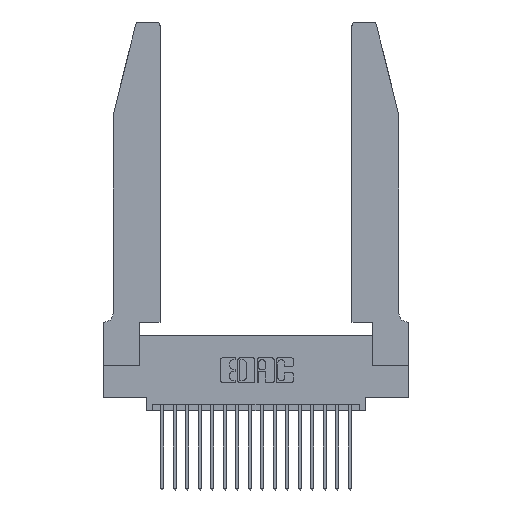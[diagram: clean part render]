
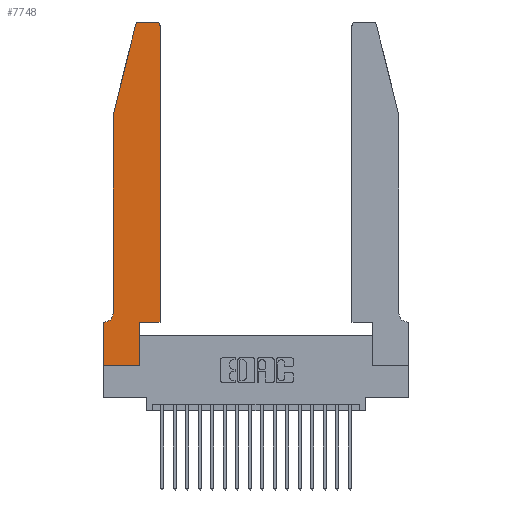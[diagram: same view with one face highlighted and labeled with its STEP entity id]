
A CAD part, top view. The second image highlights one B-rep face of the part: STEP entity #7748.
In plain terms, the highlighted planar face has unit normal (0, 0, 1).
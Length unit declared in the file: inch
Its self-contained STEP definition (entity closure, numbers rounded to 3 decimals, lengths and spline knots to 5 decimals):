
#92 = CARTESIAN_POINT ( 'NONE',  ( 0.2605, 2.75, 0.37 ) ) ;
#198 = DIRECTION ( 'NONE',  ( -1., 0., 0. ) ) ;
#615 = CARTESIAN_POINT ( 'NONE',  ( 0.4505, 0.35, 0.37 ) ) ;
#649 = ORIENTED_EDGE ( 'NONE', *, *, #16710, .T. ) ;
#1823 = VERTEX_POINT ( 'NONE', #10406 ) ;
#1873 = VERTEX_POINT ( 'NONE', #13805 ) ;
#2402 = VERTEX_POINT ( 'NONE', #5534 ) ;
#2595 = CARTESIAN_POINT ( 'NONE',  ( 0.25487, 2.72718, 0.37 ) ) ;
#2842 = DIRECTION ( 'NONE',  ( 0., 0., 1. ) ) ;
#2974 = CARTESIAN_POINT ( 'NONE',  ( 0., 0., 0.37 ) ) ;
#3159 = EDGE_CURVE ( 'NONE', #13457, #8409, #9979, .T. ) ;
#3183 = CARTESIAN_POINT ( 'NONE',  ( 0.0055, 0.35, 0.37 ) ) ;
#3323 = FACE_OUTER_BOUND ( 'NONE', #18775, .T. ) ;
#3394 = LINE ( 'NONE', #15397, #6184 ) ;
#3565 = CIRCLE ( 'NONE', #10356, 0.07 ) ;
#3956 = DIRECTION ( 'NONE',  ( 0., 1., 0. ) ) ;
#4729 = VERTEX_POINT ( 'NONE', #3183 ) ;
#5154 = EDGE_CURVE ( 'NONE', #2402, #15392, #16487, .T. ) ;
#5311 = EDGE_CURVE ( 'NONE', #18256, #2402, #11683, .T. ) ;
#5534 = CARTESIAN_POINT ( 'NONE',  ( 0.284, 2.75, 0.37 ) ) ;
#6184 = VECTOR ( 'NONE', #3956, 39.37008 ) ;
#6278 = DIRECTION ( 'NONE',  ( 0., 0., 1. ) ) ;
#6350 = CARTESIAN_POINT ( 'NONE',  ( 0.284, 2.72, 0.37 ) ) ;
#6477 = ORIENTED_EDGE ( 'NONE', *, *, #20467, .T. ) ;
#6614 = EDGE_CURVE ( 'NONE', #8911, #20233, #6688, .T. ) ;
#6688 = LINE ( 'NONE', #12629, #11731 ) ;
#6787 = ORIENTED_EDGE ( 'NONE', *, *, #10828, .T. ) ;
#7093 = CARTESIAN_POINT ( 'NONE',  ( 0.4205, 2.72, 0.37 ) ) ;
#7231 = CARTESIAN_POINT ( 'NONE',  ( 0.4205, 2.75, 0.37 ) ) ;
#7325 = DIRECTION ( 'NONE',  ( -1., 0., 0. ) ) ;
#7343 = EDGE_CURVE ( 'NONE', #20233, #1823, #18026, .T. ) ;
#7470 = ORIENTED_EDGE ( 'NONE', *, *, #7343, .T. ) ;
#7748 = ADVANCED_FACE ( 'NONE', ( #3323 ), #11911, .T. ) ;
#7940 = VECTOR ( 'NONE', #198, 39.37008 ) ;
#8409 = VERTEX_POINT ( 'NONE', #8895 ) ;
#8895 = CARTESIAN_POINT ( 'NONE',  ( 0.0755, 0.42, 0.37 ) ) ;
#8911 = VERTEX_POINT ( 'NONE', #19787 ) ;
#9188 = DIRECTION ( 'NONE',  ( 1., 0., 0. ) ) ;
#9719 = ORIENTED_EDGE ( 'NONE', *, *, #6614, .T. ) ;
#9979 = LINE ( 'NONE', #15523, #20868 ) ;
#10356 = AXIS2_PLACEMENT_3D ( 'NONE', #20347, #12143, #7325 ) ;
#10406 = CARTESIAN_POINT ( 'NONE',  ( 0.2865, 0., 0.37 ) ) ;
#10728 = DIRECTION ( 'NONE',  ( 0., -1., 0. ) ) ;
#10732 = VERTEX_POINT ( 'NONE', #17346 ) ;
#10793 = EDGE_CURVE ( 'NONE', #1873, #18256, #17385, .T. ) ;
#10828 = EDGE_CURVE ( 'NONE', #1823, #10732, #19160, .T. ) ;
#11485 = ORIENTED_EDGE ( 'NONE', *, *, #5311, .T. ) ;
#11492 = DIRECTION ( 'NONE',  ( -1., 0., 0. ) ) ;
#11619 = ORIENTED_EDGE ( 'NONE', *, *, #14231, .T. ) ;
#11683 = LINE ( 'NONE', #92, #18528 ) ;
#11731 = VECTOR ( 'NONE', #16290, 39.37008 ) ;
#11852 = AXIS2_PLACEMENT_3D ( 'NONE', #16579, #2842, #9188 ) ;
#11896 = DIRECTION ( 'NONE',  ( 1., 0., 0. ) ) ;
#11911 = PLANE ( 'NONE',  #11852 ) ;
#12005 = DIRECTION ( 'NONE',  ( 1., 0., 0. ) ) ;
#12143 = DIRECTION ( 'NONE',  ( 0., 0., -1. ) ) ;
#12629 = CARTESIAN_POINT ( 'NONE',  ( 0., 0., 0.37 ) ) ;
#13005 = CARTESIAN_POINT ( 'NONE',  ( 0.4505, 0.35, 0.37 ) ) ;
#13352 = CARTESIAN_POINT ( 'NONE',  ( 0.0755, 2., 0.37 ) ) ;
#13457 = VERTEX_POINT ( 'NONE', #16634 ) ;
#13805 = CARTESIAN_POINT ( 'NONE',  ( 0.4505, 2.72, 0.37 ) ) ;
#13833 = VECTOR ( 'NONE', #18332, 39.37008 ) ;
#14231 = EDGE_CURVE ( 'NONE', #15392, #13457, #19196, .T. ) ;
#14837 = CARTESIAN_POINT ( 'NONE',  ( 0.0755, 0.35, 0.37 ) ) ;
#15274 = ORIENTED_EDGE ( 'NONE', *, *, #10793, .T. ) ;
#15392 = VERTEX_POINT ( 'NONE', #2595 ) ;
#15397 = CARTESIAN_POINT ( 'NONE',  ( 0.4505, 0.35, 0.37 ) ) ;
#15523 = CARTESIAN_POINT ( 'NONE',  ( 0.0755, 2., 0.37 ) ) ;
#15713 = CARTESIAN_POINT ( 'NONE',  ( 0., 0., 0.37 ) ) ;
#16290 = DIRECTION ( 'NONE',  ( 0., -1., 0. ) ) ;
#16487 = CIRCLE ( 'NONE', #16822, 0.03 ) ;
#16579 = CARTESIAN_POINT ( 'NONE',  ( 0., 0.35, 0.37 ) ) ;
#16634 = CARTESIAN_POINT ( 'NONE',  ( 0.0755, 2., 0.37 ) ) ;
#16701 = CARTESIAN_POINT ( 'NONE',  ( 0.2865, 0.35, 0.37 ) ) ;
#16710 = EDGE_CURVE ( 'NONE', #10732, #19386, #18593, .T. ) ;
#16822 = AXIS2_PLACEMENT_3D ( 'NONE', #6350, #6278, #17587 ) ;
#17293 = LINE ( 'NONE', #14837, #7940 ) ;
#17346 = CARTESIAN_POINT ( 'NONE',  ( 0.2865, 0.35, 0.37 ) ) ;
#17385 = CIRCLE ( 'NONE', #20580, 0.03 ) ;
#17531 = EDGE_CURVE ( 'NONE', #4729, #8911, #17293, .T. ) ;
#17587 = DIRECTION ( 'NONE',  ( 1., 0., 0. ) ) ;
#17596 = DIRECTION ( 'NONE',  ( -0.239, -0.971, 0. ) ) ;
#17795 = ORIENTED_EDGE ( 'NONE', *, *, #19012, .T. ) ;
#18026 = LINE ( 'NONE', #15713, #20314 ) ;
#18256 = VERTEX_POINT ( 'NONE', #7231 ) ;
#18332 = DIRECTION ( 'NONE',  ( 0., 1., 0. ) ) ;
#18348 = ORIENTED_EDGE ( 'NONE', *, *, #5154, .T. ) ;
#18404 = DIRECTION ( 'NONE',  ( 0., 0., 1. ) ) ;
#18528 = VECTOR ( 'NONE', #11492, 39.37008 ) ;
#18593 = LINE ( 'NONE', #615, #20642 ) ;
#18775 = EDGE_LOOP ( 'NONE', ( #11485, #18348, #11619, #20822, #6477, #19100, #9719, #7470, #6787, #649, #17795, #15274 ) ) ;
#19012 = EDGE_CURVE ( 'NONE', #19386, #1873, #3394, .T. ) ;
#19100 = ORIENTED_EDGE ( 'NONE', *, *, #17531, .T. ) ;
#19160 = LINE ( 'NONE', #16701, #13833 ) ;
#19196 = LINE ( 'NONE', #13352, #19711 ) ;
#19386 = VERTEX_POINT ( 'NONE', #13005 ) ;
#19711 = VECTOR ( 'NONE', #17596, 39.37008 ) ;
#19787 = CARTESIAN_POINT ( 'NONE',  ( 0., 0.35, 0.37 ) ) ;
#19986 = DIRECTION ( 'NONE',  ( 1., 0., 0. ) ) ;
#20233 = VERTEX_POINT ( 'NONE', #2974 ) ;
#20314 = VECTOR ( 'NONE', #11896, 39.37008 ) ;
#20347 = CARTESIAN_POINT ( 'NONE',  ( 0.0055, 0.42, 0.37 ) ) ;
#20467 = EDGE_CURVE ( 'NONE', #8409, #4729, #3565, .T. ) ;
#20580 = AXIS2_PLACEMENT_3D ( 'NONE', #7093, #18404, #19986 ) ;
#20642 = VECTOR ( 'NONE', #12005, 39.37008 ) ;
#20822 = ORIENTED_EDGE ( 'NONE', *, *, #3159, .T. ) ;
#20868 = VECTOR ( 'NONE', #10728, 39.37008 ) ;
